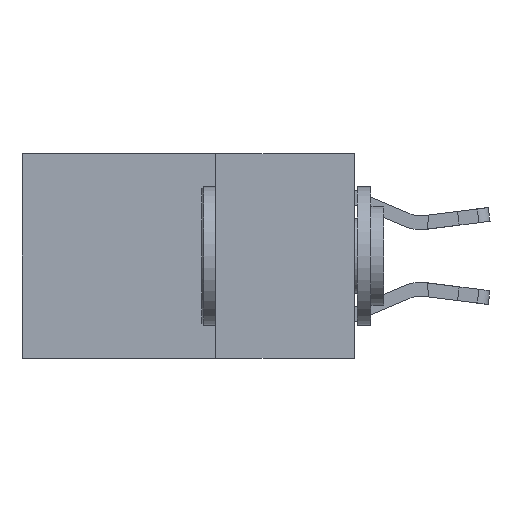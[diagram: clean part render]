
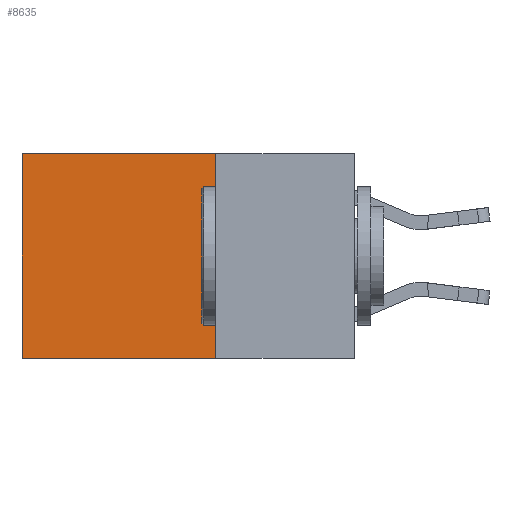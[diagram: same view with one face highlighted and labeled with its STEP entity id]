
A CAD part, left-side view. The second image highlights one B-rep face of the part: STEP entity #8635.
In plain terms, the highlighted planar face has unit normal (-1, 0, 0).
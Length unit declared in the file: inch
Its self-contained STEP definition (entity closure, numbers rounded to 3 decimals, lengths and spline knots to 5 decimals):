
#234 = ORIENTED_EDGE ( 'NONE', *, *, #8549, .F. ) ;
#1658 = CARTESIAN_POINT ( 'NONE',  ( 0.2625, 0.6, 0. ) ) ;
#1719 = EDGE_CURVE ( 'NONE', #10925, #12205, #6798, .T. ) ;
#1791 = LINE ( 'NONE', #12293, #8409 ) ;
#2068 = FACE_OUTER_BOUND ( 'NONE', #7693, .T. ) ;
#2125 = LINE ( 'NONE', #7253, #7280 ) ;
#2662 = DIRECTION ( 'NONE',  ( 1., 0., 0. ) ) ;
#2747 = DIRECTION ( 'NONE',  ( 0., 0., -1. ) ) ;
#3549 = DIRECTION ( 'NONE',  ( 0., 1., 0. ) ) ;
#3847 = ORIENTED_EDGE ( 'NONE', *, *, #7408, .F. ) ;
#4358 = DIRECTION ( 'NONE',  ( 0., 0., -1. ) ) ;
#4512 = VERTEX_POINT ( 'NONE', #12116 ) ;
#4709 = AXIS2_PLACEMENT_3D ( 'NONE', #11602, #2662, #9846 ) ;
#4795 = CARTESIAN_POINT ( 'NONE',  ( 0.2625, 0.6, 0. ) ) ;
#4897 = EDGE_CURVE ( 'NONE', #10234, #10925, #1791, .T. ) ;
#5615 = CARTESIAN_POINT ( 'NONE',  ( 0.2625, 0.6, -0.37 ) ) ;
#6177 = PLANE ( 'NONE',  #4709 ) ;
#6798 = LINE ( 'NONE', #1658, #7647 ) ;
#7253 = CARTESIAN_POINT ( 'NONE',  ( 0.2625, 0.25, 0. ) ) ;
#7280 = VECTOR ( 'NONE', #4358, 39.37008 ) ;
#7408 = EDGE_CURVE ( 'NONE', #4512, #12205, #7637, .T. ) ;
#7442 = CARTESIAN_POINT ( 'NONE',  ( 0.2625, 0.25, 0. ) ) ;
#7586 = VECTOR ( 'NONE', #3549, 39.37008 ) ;
#7637 = LINE ( 'NONE', #10520, #7586 ) ;
#7647 = VECTOR ( 'NONE', #2747, 39.37008 ) ;
#7693 = EDGE_LOOP ( 'NONE', ( #11092, #3847, #234, #11970 ) ) ;
#8409 = VECTOR ( 'NONE', #12224, 39.37008 ) ;
#8549 = EDGE_CURVE ( 'NONE', #10234, #4512, #2125, .T. ) ;
#8635 = ADVANCED_FACE ( 'NONE', ( #2068 ), #6177, .F. ) ;
#9846 = DIRECTION ( 'NONE',  ( 0., 0., -1. ) ) ;
#10234 = VERTEX_POINT ( 'NONE', #7442 ) ;
#10520 = CARTESIAN_POINT ( 'NONE',  ( 0.2625, 0.25, -0.37 ) ) ;
#10925 = VERTEX_POINT ( 'NONE', #4795 ) ;
#11092 = ORIENTED_EDGE ( 'NONE', *, *, #1719, .T. ) ;
#11602 = CARTESIAN_POINT ( 'NONE',  ( 0.2625, 0.25, 0. ) ) ;
#11970 = ORIENTED_EDGE ( 'NONE', *, *, #4897, .T. ) ;
#12116 = CARTESIAN_POINT ( 'NONE',  ( 0.2625, 0.25, -0.37 ) ) ;
#12205 = VERTEX_POINT ( 'NONE', #5615 ) ;
#12224 = DIRECTION ( 'NONE',  ( 0., 1., 0. ) ) ;
#12293 = CARTESIAN_POINT ( 'NONE',  ( 0.2625, 0.25, 0. ) ) ;
